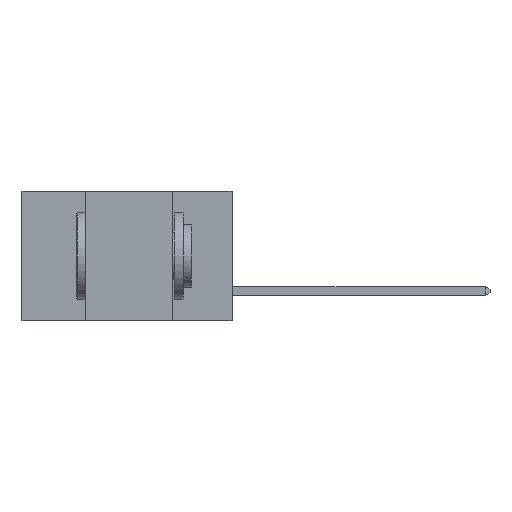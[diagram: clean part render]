
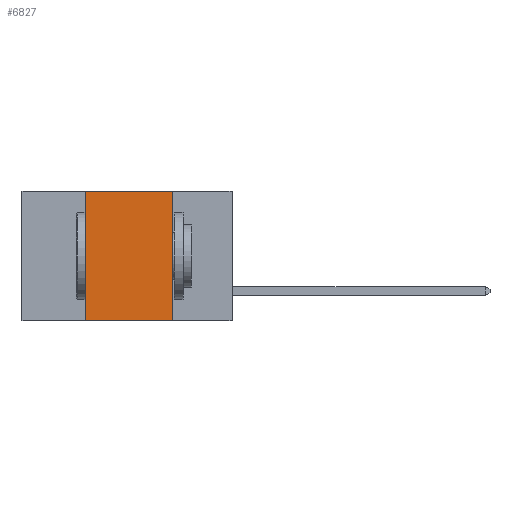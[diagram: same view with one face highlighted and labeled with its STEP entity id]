
A CAD part, left-side view. The second image highlights one B-rep face of the part: STEP entity #6827.
In plain terms, the highlighted planar face has unit normal (-1, 0, 0).
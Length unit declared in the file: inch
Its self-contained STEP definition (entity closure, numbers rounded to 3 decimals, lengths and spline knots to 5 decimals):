
#988 = DIRECTION ( 'NONE',  ( 0., -1., 0. ) ) ;
#1128 = CARTESIAN_POINT ( 'NONE',  ( 0., 0.6, -0.37 ) ) ;
#1818 = CARTESIAN_POINT ( 'NONE',  ( 0., 0.42, 0. ) ) ;
#2994 = EDGE_LOOP ( 'NONE', ( #15107, #15486, #15592, #15707 ) ) ;
#3792 = EDGE_CURVE ( 'NONE', #13900, #6665, #19636, .T. ) ;
#4257 = VECTOR ( 'NONE', #11100, 39.37008 ) ;
#5583 = EDGE_CURVE ( 'NONE', #10024, #18648, #24077, .T. ) ;
#6665 = VERTEX_POINT ( 'NONE', #14141 ) ;
#6827 = ADVANCED_FACE ( 'NONE', ( #9348 ), #20924, .F. ) ;
#7640 = DIRECTION ( 'NONE',  ( 0., 0., 1. ) ) ;
#9348 = FACE_OUTER_BOUND ( 'NONE', #2994, .T. ) ;
#10024 = VERTEX_POINT ( 'NONE', #1818 ) ;
#10916 = EDGE_CURVE ( 'NONE', #13900, #10024, #23692, .T. ) ;
#11100 = DIRECTION ( 'NONE',  ( 0., 0., -1. ) ) ;
#11541 = VECTOR ( 'NONE', #7640, 39.37008 ) ;
#11761 = DIRECTION ( 'NONE',  ( 0., 0., -1. ) ) ;
#12644 = DIRECTION ( 'NONE',  ( 0., -1., 0. ) ) ;
#13484 = VECTOR ( 'NONE', #988, 39.37008 ) ;
#13900 = VERTEX_POINT ( 'NONE', #20841 ) ;
#14141 = CARTESIAN_POINT ( 'NONE',  ( 0., 0.17, -0.37 ) ) ;
#15107 = ORIENTED_EDGE ( 'NONE', *, *, #18681, .F. ) ;
#15265 = AXIS2_PLACEMENT_3D ( 'NONE', #23174, #25499, #11761 ) ;
#15486 = ORIENTED_EDGE ( 'NONE', *, *, #5583, .F. ) ;
#15592 = ORIENTED_EDGE ( 'NONE', *, *, #10916, .F. ) ;
#15707 = ORIENTED_EDGE ( 'NONE', *, *, #3792, .T. ) ;
#16633 = LINE ( 'NONE', #20263, #4257 ) ;
#17354 = VECTOR ( 'NONE', #12644, 39.37008 ) ;
#18648 = VERTEX_POINT ( 'NONE', #26881 ) ;
#18681 = EDGE_CURVE ( 'NONE', #18648, #6665, #16633, .T. ) ;
#19636 = LINE ( 'NONE', #1128, #13484 ) ;
#20263 = CARTESIAN_POINT ( 'NONE',  ( 0., 0.17, 0. ) ) ;
#20841 = CARTESIAN_POINT ( 'NONE',  ( 0., 0.42, -0.37 ) ) ;
#20924 = PLANE ( 'NONE',  #15265 ) ;
#23174 = CARTESIAN_POINT ( 'NONE',  ( 0., 0.6, 0. ) ) ;
#23687 = CARTESIAN_POINT ( 'NONE',  ( 0., 0.42, 0. ) ) ;
#23692 = LINE ( 'NONE', #23687, #11541 ) ;
#24054 = CARTESIAN_POINT ( 'NONE',  ( 0., 0.6, 0. ) ) ;
#24077 = LINE ( 'NONE', #24054, #17354 ) ;
#25499 = DIRECTION ( 'NONE',  ( 1., 0., 0. ) ) ;
#26881 = CARTESIAN_POINT ( 'NONE',  ( 0., 0.17, 0. ) ) ;
